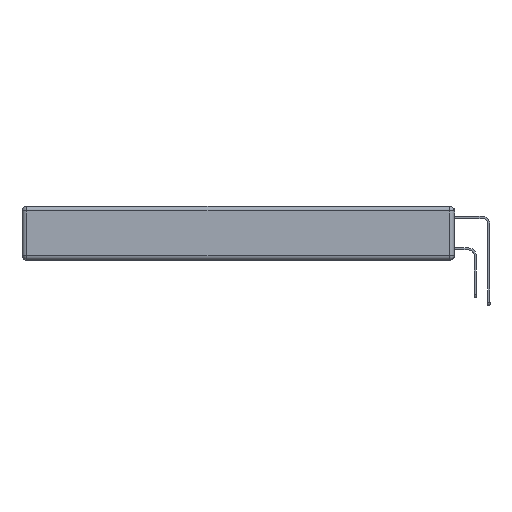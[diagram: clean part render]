
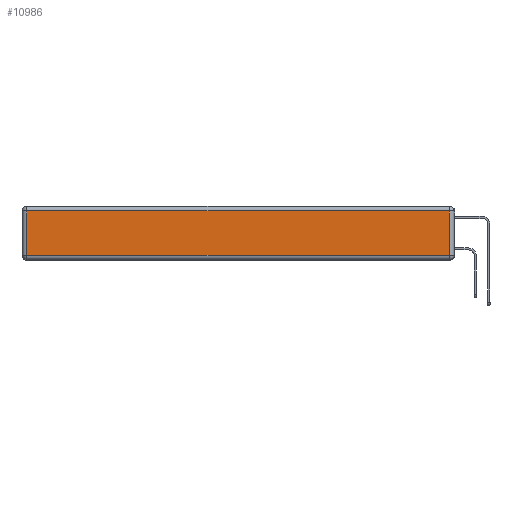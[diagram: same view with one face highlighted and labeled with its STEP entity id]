
A CAD part, left-side view. The second image highlights one B-rep face of the part: STEP entity #10986.
In plain terms, the highlighted planar face has unit normal (-1, 0, 0).
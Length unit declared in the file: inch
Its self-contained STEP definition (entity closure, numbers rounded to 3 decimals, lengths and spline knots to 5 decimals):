
#102 = VECTOR ( 'NONE', #5452, 39.37008 ) ;
#1055 = VERTEX_POINT ( 'NONE', #17359 ) ;
#1878 = VERTEX_POINT ( 'NONE', #3276 ) ;
#2089 = ORIENTED_EDGE ( 'NONE', *, *, #16666, .T. ) ;
#2856 = CARTESIAN_POINT ( 'NONE',  ( 0., 2.72, -0.343 ) ) ;
#3043 = VERTEX_POINT ( 'NONE', #10056 ) ;
#3276 = CARTESIAN_POINT ( 'NONE',  ( 0., 0.03, -0.313 ) ) ;
#3284 = PLANE ( 'NONE',  #11029 ) ;
#4112 = EDGE_CURVE ( 'NONE', #1055, #3043, #10291, .T. ) ;
#4806 = DIRECTION ( 'NONE',  ( -1., 0., 0. ) ) ;
#5203 = LINE ( 'NONE', #12087, #17048 ) ;
#5217 = CARTESIAN_POINT ( 'NONE',  ( 0., 0., -0.343 ) ) ;
#5452 = DIRECTION ( 'NONE',  ( 0., 1., 0. ) ) ;
#5706 = LINE ( 'NONE', #18497, #15506 ) ;
#8053 = EDGE_LOOP ( 'NONE', ( #2089, #12846, #18067, #11674 ) ) ;
#10056 = CARTESIAN_POINT ( 'NONE',  ( 0., 2.72, -0.313 ) ) ;
#10291 = LINE ( 'NONE', #2856, #18201 ) ;
#10986 = ADVANCED_FACE ( 'NONE', ( #18203 ), #3284, .T. ) ;
#11029 = AXIS2_PLACEMENT_3D ( 'NONE', #5217, #4806, #16709 ) ;
#11434 = CARTESIAN_POINT ( 'NONE',  ( 0., 0.03, -0.03 ) ) ;
#11674 = ORIENTED_EDGE ( 'NONE', *, *, #4112, .T. ) ;
#12087 = CARTESIAN_POINT ( 'NONE',  ( 0., 0., -0.313 ) ) ;
#12846 = ORIENTED_EDGE ( 'NONE', *, *, #15836, .T. ) ;
#13637 = CARTESIAN_POINT ( 'NONE',  ( 0., 2.75, -0.03 ) ) ;
#13887 = EDGE_CURVE ( 'NONE', #14566, #1055, #16746, .T. ) ;
#14189 = DIRECTION ( 'NONE',  ( 0., 0., 1. ) ) ;
#14566 = VERTEX_POINT ( 'NONE', #11434 ) ;
#15506 = VECTOR ( 'NONE', #14189, 39.37008 ) ;
#15836 = EDGE_CURVE ( 'NONE', #1878, #14566, #5706, .T. ) ;
#16666 = EDGE_CURVE ( 'NONE', #3043, #1878, #5203, .T. ) ;
#16695 = DIRECTION ( 'NONE',  ( 0., -1., 0. ) ) ;
#16709 = DIRECTION ( 'NONE',  ( 0., 0., 1. ) ) ;
#16746 = LINE ( 'NONE', #13637, #102 ) ;
#17048 = VECTOR ( 'NONE', #16695, 39.37008 ) ;
#17359 = CARTESIAN_POINT ( 'NONE',  ( 0., 2.72, -0.03 ) ) ;
#17462 = DIRECTION ( 'NONE',  ( 0., 0., -1. ) ) ;
#18067 = ORIENTED_EDGE ( 'NONE', *, *, #13887, .T. ) ;
#18201 = VECTOR ( 'NONE', #17462, 39.37008 ) ;
#18203 = FACE_OUTER_BOUND ( 'NONE', #8053, .T. ) ;
#18497 = CARTESIAN_POINT ( 'NONE',  ( 0., 0.03, -0.343 ) ) ;
